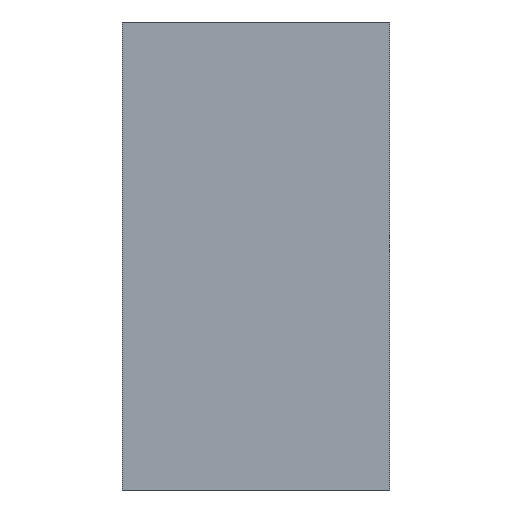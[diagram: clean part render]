
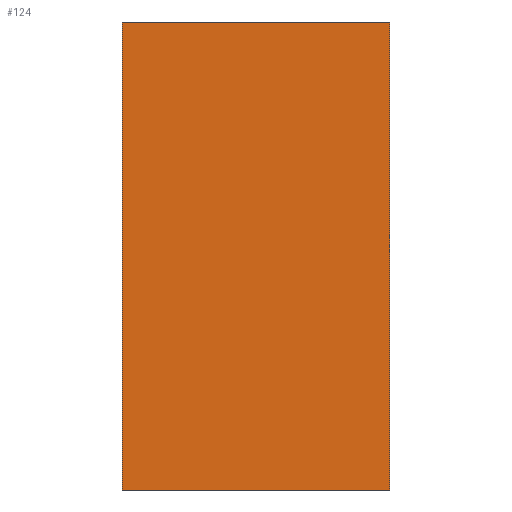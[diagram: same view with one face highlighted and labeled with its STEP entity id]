
A CAD part, left-side view. The second image highlights one B-rep face of the part: STEP entity #124.
In plain terms, the highlighted planar face has unit normal (-1, 0, 0).
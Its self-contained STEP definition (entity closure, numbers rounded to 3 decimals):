
#24=FACE_OUTER_BOUND('',#33,.T.);
#33=EDGE_LOOP('',(#95,#96,#97,#98));
#39=LINE('',#197,#50);
#43=LINE('',#207,#54);
#45=LINE('',#213,#56);
#46=LINE('',#214,#57);
#50=VECTOR('',#160,10.);
#54=VECTOR('',#168,10.);
#56=VECTOR('',#174,10.);
#57=VECTOR('',#175,10.);
#61=VERTEX_POINT('',#195);
#62=VERTEX_POINT('',#196);
#66=VERTEX_POINT('',#206);
#68=VERTEX_POINT('',#212);
#71=EDGE_CURVE('',#61,#62,#39,.T.);
#76=EDGE_CURVE('',#61,#66,#43,.T.);
#79=EDGE_CURVE('',#62,#68,#45,.T.);
#80=EDGE_CURVE('',#66,#68,#46,.T.);
#95=ORIENTED_EDGE('',*,*,#71,.T.);
#96=ORIENTED_EDGE('',*,*,#79,.T.);
#97=ORIENTED_EDGE('',*,*,#80,.F.);
#98=ORIENTED_EDGE('',*,*,#76,.F.);
#118=PLANE('',#148);
#124=ADVANCED_FACE('',(#24),#118,.T.);
#148=AXIS2_PLACEMENT_3D('',#211,#172,#173);
#160=DIRECTION('',(0.,0.,1.));
#168=DIRECTION('',(0.,1.,0.));
#172=DIRECTION('center_axis',(-1.,0.,0.));
#173=DIRECTION('ref_axis',(0.,0.,1.));
#174=DIRECTION('',(0.,1.,0.));
#175=DIRECTION('',(0.,0.,1.));
#195=CARTESIAN_POINT('',(0.,1.,-7.));
#196=CARTESIAN_POINT('',(0.,1.,0.));
#197=CARTESIAN_POINT('',(0.,1.,-5.25));
#206=CARTESIAN_POINT('',(0.,5.,-7.));
#207=CARTESIAN_POINT('',(0.,0.,-7.));
#211=CARTESIAN_POINT('Origin',(0.,0.,-7.));
#212=CARTESIAN_POINT('',(0.,5.,0.));
#213=CARTESIAN_POINT('',(0.,0.,0.));
#214=CARTESIAN_POINT('',(0.,5.,-7.));
